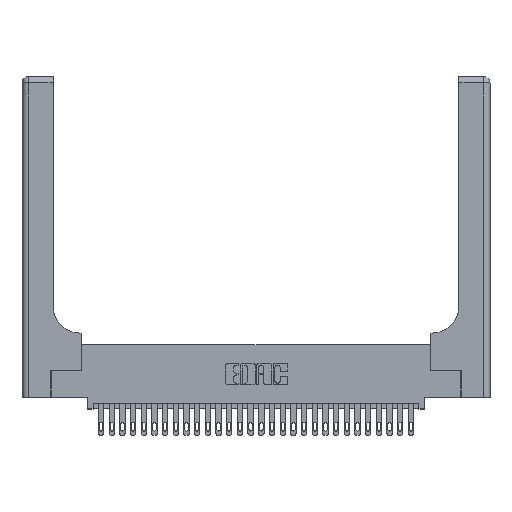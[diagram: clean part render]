
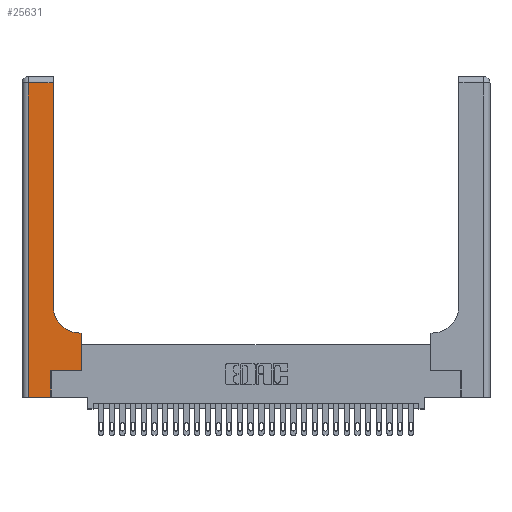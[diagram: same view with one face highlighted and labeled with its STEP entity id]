
A CAD part, top view. The second image highlights one B-rep face of the part: STEP entity #25631.
In plain terms, the highlighted planar face has unit normal (0, 0, 1).
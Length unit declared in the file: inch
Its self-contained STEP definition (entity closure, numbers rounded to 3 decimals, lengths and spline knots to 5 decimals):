
#297 = ORIENTED_EDGE ( 'NONE', *, *, #27711, .T. ) ;
#486 = EDGE_CURVE ( 'NONE', #8911, #25531, #4602, .T. ) ;
#1514 = ORIENTED_EDGE ( 'NONE', *, *, #8132, .T. ) ;
#1677 = DIRECTION ( 'NONE',  ( 1., 0., 0. ) ) ;
#1916 = DIRECTION ( 'NONE',  ( 0., 1., 0. ) ) ;
#2134 = EDGE_CURVE ( 'NONE', #6749, #8911, #10465, .T. ) ;
#2414 = EDGE_CURVE ( 'NONE', #25531, #17396, #22904, .T. ) ;
#3106 = AXIS2_PLACEMENT_3D ( 'NONE', #23251, #16382, #16188 ) ;
#3277 = VECTOR ( 'NONE', #22438, 39.37008 ) ;
#3290 = CARTESIAN_POINT ( 'NONE',  ( 0.269, 0., 0.37 ) ) ;
#4191 = CARTESIAN_POINT ( 'NONE',  ( 0.06, 2.94, 0.37 ) ) ;
#4602 = LINE ( 'NONE', #4950, #4951 ) ;
#4678 = EDGE_LOOP ( 'NONE', ( #297, #27974, #18542, #14562, #9158, #19962, #1514, #24616, #17896 ) ) ;
#4950 = CARTESIAN_POINT ( 'NONE',  ( 0., 0., 0.37 ) ) ;
#4951 = VECTOR ( 'NONE', #21361, 39.37008 ) ;
#4965 = VECTOR ( 'NONE', #13689, 39.37008 ) ;
#5476 = CARTESIAN_POINT ( 'NONE',  ( 0.2915, 2.94, 0.37 ) ) ;
#5694 = LINE ( 'NONE', #9149, #4965 ) ;
#6091 = CARTESIAN_POINT ( 'NONE',  ( 0.2915, 3., 0.37 ) ) ;
#6303 = VECTOR ( 'NONE', #1916, 39.37008 ) ;
#6749 = VERTEX_POINT ( 'NONE', #4191 ) ;
#8132 = EDGE_CURVE ( 'NONE', #12214, #22218, #15784, .T. ) ;
#8183 = VERTEX_POINT ( 'NONE', #8390 ) ;
#8307 = DIRECTION ( 'NONE',  ( 0., 1., 0. ) ) ;
#8390 = CARTESIAN_POINT ( 'NONE',  ( 0.2915, 0.85, 0.37 ) ) ;
#8911 = VERTEX_POINT ( 'NONE', #25702 ) ;
#9149 = CARTESIAN_POINT ( 'NONE',  ( 0.2915, 0.6, 0.37 ) ) ;
#9158 = ORIENTED_EDGE ( 'NONE', *, *, #2414, .T. ) ;
#9583 = CARTESIAN_POINT ( 'NONE',  ( 0.06, 3., 0.37 ) ) ;
#9958 = CARTESIAN_POINT ( 'NONE',  ( 0.5415, 0.6, 0.37 ) ) ;
#10465 = LINE ( 'NONE', #9583, #28069 ) ;
#10564 = DIRECTION ( 'NONE',  ( -1., 0., 0. ) ) ;
#10723 = VERTEX_POINT ( 'NONE', #9958 ) ;
#11004 = CARTESIAN_POINT ( 'NONE',  ( 0.5415, 0.85, 0.37 ) ) ;
#11083 = FACE_OUTER_BOUND ( 'NONE', #4678, .T. ) ;
#11508 = LINE ( 'NONE', #6091, #6303 ) ;
#12214 = VERTEX_POINT ( 'NONE', #23307 ) ;
#12940 = LINE ( 'NONE', #27056, #24269 ) ;
#13374 = AXIS2_PLACEMENT_3D ( 'NONE', #11004, #18281, #1677 ) ;
#13689 = DIRECTION ( 'NONE',  ( -1., 0., 0. ) ) ;
#14014 = DIRECTION ( 'NONE',  ( 0., -1., 0. ) ) ;
#14562 = ORIENTED_EDGE ( 'NONE', *, *, #486, .T. ) ;
#14582 = CIRCLE ( 'NONE', #13374, 0.25 ) ;
#15784 = LINE ( 'NONE', #29221, #3277 ) ;
#16100 = CARTESIAN_POINT ( 'NONE',  ( 0.269, 0.25, 0.37 ) ) ;
#16188 = DIRECTION ( 'NONE',  ( -1., 0., 0. ) ) ;
#16336 = VERTEX_POINT ( 'NONE', #5476 ) ;
#16382 = DIRECTION ( 'NONE',  ( 0., 0., -1. ) ) ;
#17396 = VERTEX_POINT ( 'NONE', #16100 ) ;
#17896 = ORIENTED_EDGE ( 'NONE', *, *, #30332, .T. ) ;
#18031 = CARTESIAN_POINT ( 'NONE',  ( 0.5585, 0.6, 0.37 ) ) ;
#18281 = DIRECTION ( 'NONE',  ( 0., 0., -1. ) ) ;
#18542 = ORIENTED_EDGE ( 'NONE', *, *, #2134, .T. ) ;
#19054 = LINE ( 'NONE', #19167, #26780 ) ;
#19167 = CARTESIAN_POINT ( 'NONE',  ( 0.269, 0.25, 0.37 ) ) ;
#19962 = ORIENTED_EDGE ( 'NONE', *, *, #28584, .T. ) ;
#20298 = CARTESIAN_POINT ( 'NONE',  ( 0.269, 0., 0.37 ) ) ;
#20700 = VECTOR ( 'NONE', #8307, 39.37008 ) ;
#21096 = PLANE ( 'NONE',  #3106 ) ;
#21361 = DIRECTION ( 'NONE',  ( 1., 0., 0. ) ) ;
#21610 = EDGE_CURVE ( 'NONE', #22218, #10723, #5694, .T. ) ;
#22218 = VERTEX_POINT ( 'NONE', #18031 ) ;
#22438 = DIRECTION ( 'NONE',  ( 0., 1., 0. ) ) ;
#22904 = LINE ( 'NONE', #3290, #20700 ) ;
#23251 = CARTESIAN_POINT ( 'NONE',  ( 0., 3., 0.37 ) ) ;
#23307 = CARTESIAN_POINT ( 'NONE',  ( 0.5585, 0.25, 0.37 ) ) ;
#24016 = DIRECTION ( 'NONE',  ( 1., 0., 0. ) ) ;
#24269 = VECTOR ( 'NONE', #10564, 39.37008 ) ;
#24616 = ORIENTED_EDGE ( 'NONE', *, *, #21610, .T. ) ;
#25497 = EDGE_CURVE ( 'NONE', #16336, #6749, #12940, .T. ) ;
#25531 = VERTEX_POINT ( 'NONE', #20298 ) ;
#25631 = ADVANCED_FACE ( 'NONE', ( #11083 ), #21096, .F. ) ;
#25702 = CARTESIAN_POINT ( 'NONE',  ( 0.06, 0., 0.37 ) ) ;
#26780 = VECTOR ( 'NONE', #24016, 39.37008 ) ;
#27056 = CARTESIAN_POINT ( 'NONE',  ( 0., 2.94, 0.37 ) ) ;
#27711 = EDGE_CURVE ( 'NONE', #8183, #16336, #11508, .T. ) ;
#27974 = ORIENTED_EDGE ( 'NONE', *, *, #25497, .T. ) ;
#28069 = VECTOR ( 'NONE', #14014, 39.37008 ) ;
#28584 = EDGE_CURVE ( 'NONE', #17396, #12214, #19054, .T. ) ;
#29221 = CARTESIAN_POINT ( 'NONE',  ( 0.5585, 0.25, 0.37 ) ) ;
#30332 = EDGE_CURVE ( 'NONE', #10723, #8183, #14582, .T. ) ;
